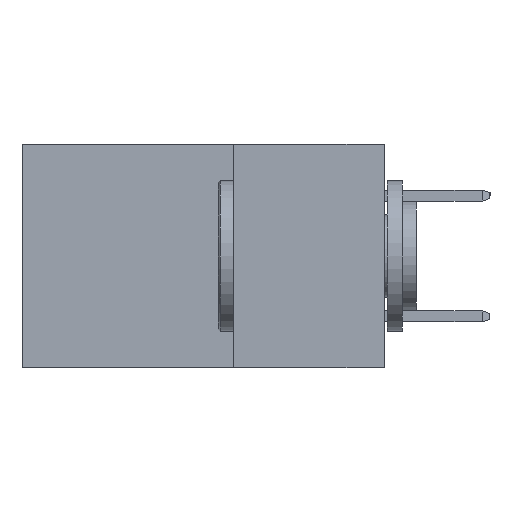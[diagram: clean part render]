
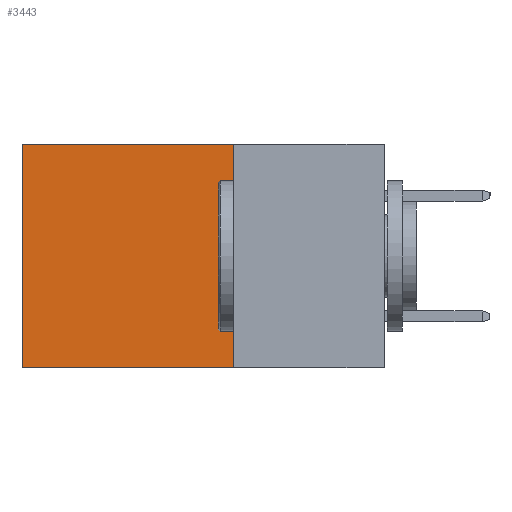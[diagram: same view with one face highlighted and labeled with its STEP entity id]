
A CAD part, left-side view. The second image highlights one B-rep face of the part: STEP entity #3443.
In plain terms, the highlighted planar face has unit normal (-1, 0, 0).
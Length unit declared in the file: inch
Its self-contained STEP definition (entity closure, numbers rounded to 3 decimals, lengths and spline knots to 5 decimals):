
#1 = VERTEX_POINT ( 'NONE', #4719 ) ;
#90 = ORIENTED_EDGE ( 'NONE', *, *, #6672, .F. ) ;
#197 = ORIENTED_EDGE ( 'NONE', *, *, #8214, .T. ) ;
#231 = EDGE_LOOP ( 'NONE', ( #6841, #90, #551, #197 ) ) ;
#551 = ORIENTED_EDGE ( 'NONE', *, *, #8255, .F. ) ;
#699 = CARTESIAN_POINT ( 'NONE',  ( 0.2615, 0.25, 0. ) ) ;
#1047 = LINE ( 'NONE', #1147, #8687 ) ;
#1147 = CARTESIAN_POINT ( 'NONE',  ( 0.2615, 0.25, -0.37 ) ) ;
#1910 = VECTOR ( 'NONE', #6559, 39.37008 ) ;
#2172 = DIRECTION ( 'NONE',  ( 0., 0., -1. ) ) ;
#2292 = VERTEX_POINT ( 'NONE', #8100 ) ;
#2422 = EDGE_CURVE ( 'NONE', #1, #4135, #3796, .T. ) ;
#3443 = ADVANCED_FACE ( 'NONE', ( #8952 ), #5958, .F. ) ;
#3796 = LINE ( 'NONE', #9031, #7625 ) ;
#4135 = VERTEX_POINT ( 'NONE', #4207 ) ;
#4207 = CARTESIAN_POINT ( 'NONE',  ( 0.2615, 0.6, -0.37 ) ) ;
#4646 = DIRECTION ( 'NONE',  ( 0., 0., -1. ) ) ;
#4719 = CARTESIAN_POINT ( 'NONE',  ( 0.2615, 0.6, 0. ) ) ;
#5036 = CARTESIAN_POINT ( 'NONE',  ( 0.2615, 0.25, 0. ) ) ;
#5092 = LINE ( 'NONE', #5036, #9493 ) ;
#5415 = CARTESIAN_POINT ( 'NONE',  ( 0.2615, 0.25, -0.37 ) ) ;
#5482 = DIRECTION ( 'NONE',  ( 0., 1., 0. ) ) ;
#5877 = CARTESIAN_POINT ( 'NONE',  ( 0.2615, 0.25, -0.37 ) ) ;
#5926 = LINE ( 'NONE', #5877, #1910 ) ;
#5958 = PLANE ( 'NONE',  #8191 ) ;
#6505 = DIRECTION ( 'NONE',  ( 0., 1., 0. ) ) ;
#6559 = DIRECTION ( 'NONE',  ( 0., 0., -1. ) ) ;
#6672 = EDGE_CURVE ( 'NONE', #2292, #4135, #1047, .T. ) ;
#6841 = ORIENTED_EDGE ( 'NONE', *, *, #2422, .T. ) ;
#7019 = VERTEX_POINT ( 'NONE', #699 ) ;
#7510 = DIRECTION ( 'NONE',  ( 1., 0., 0. ) ) ;
#7625 = VECTOR ( 'NONE', #4646, 39.37008 ) ;
#8100 = CARTESIAN_POINT ( 'NONE',  ( 0.2615, 0.25, -0.37 ) ) ;
#8191 = AXIS2_PLACEMENT_3D ( 'NONE', #5415, #7510, #2172 ) ;
#8214 = EDGE_CURVE ( 'NONE', #7019, #1, #5092, .T. ) ;
#8255 = EDGE_CURVE ( 'NONE', #7019, #2292, #5926, .T. ) ;
#8687 = VECTOR ( 'NONE', #5482, 39.37008 ) ;
#8952 = FACE_OUTER_BOUND ( 'NONE', #231, .T. ) ;
#9031 = CARTESIAN_POINT ( 'NONE',  ( 0.2615, 0.6, -0.37 ) ) ;
#9493 = VECTOR ( 'NONE', #6505, 39.37008 ) ;
